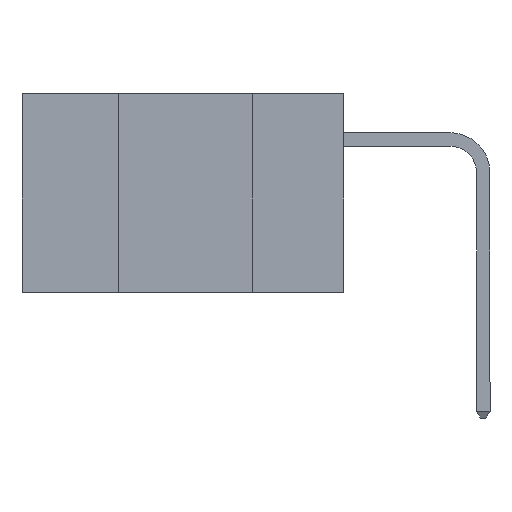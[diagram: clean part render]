
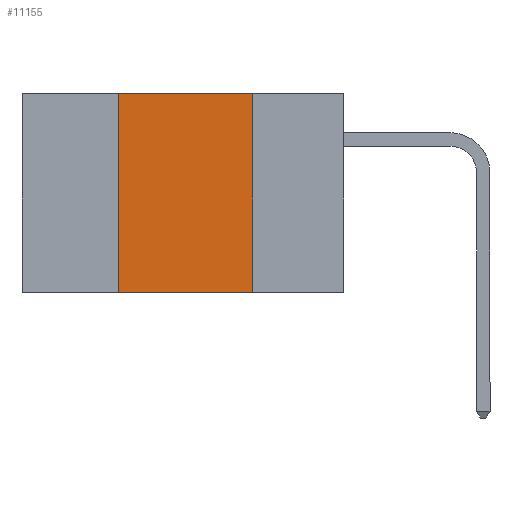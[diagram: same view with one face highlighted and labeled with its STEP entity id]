
A CAD part, left-side view. The second image highlights one B-rep face of the part: STEP entity #11155.
In plain terms, the highlighted planar face has unit normal (-1, 0, 0).
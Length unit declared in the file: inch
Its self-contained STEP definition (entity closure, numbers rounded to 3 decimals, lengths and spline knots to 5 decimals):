
#25 = VECTOR ( 'NONE', #2915, 39.37008 ) ;
#206 = ORIENTED_EDGE ( 'NONE', *, *, #9290, .T. ) ;
#364 = CARTESIAN_POINT ( 'NONE',  ( 0., 0.42, -0.37 ) ) ;
#1461 = DIRECTION ( 'NONE',  ( 0., 0., 1. ) ) ;
#1972 = PLANE ( 'NONE',  #8002 ) ;
#2119 = CARTESIAN_POINT ( 'NONE',  ( 0., 0.42, 0. ) ) ;
#2573 = LINE ( 'NONE', #13075, #5577 ) ;
#2915 = DIRECTION ( 'NONE',  ( 0., 0., -1. ) ) ;
#3255 = DIRECTION ( 'NONE',  ( 1., 0., 0. ) ) ;
#3504 = FACE_OUTER_BOUND ( 'NONE', #11073, .T. ) ;
#3637 = ORIENTED_EDGE ( 'NONE', *, *, #10864, .F. ) ;
#4754 = ORIENTED_EDGE ( 'NONE', *, *, #11659, .F. ) ;
#5577 = VECTOR ( 'NONE', #15518, 39.37008 ) ;
#8002 = AXIS2_PLACEMENT_3D ( 'NONE', #10752, #3255, #11915 ) ;
#8696 = VERTEX_POINT ( 'NONE', #364 ) ;
#9224 = CARTESIAN_POINT ( 'NONE',  ( 0., 0.17, 0. ) ) ;
#9290 = EDGE_CURVE ( 'NONE', #8696, #14213, #11735, .T. ) ;
#9798 = LINE ( 'NONE', #9224, #25 ) ;
#9907 = VERTEX_POINT ( 'NONE', #10927 ) ;
#10333 = ORIENTED_EDGE ( 'NONE', *, *, #14734, .F. ) ;
#10388 = VECTOR ( 'NONE', #1461, 39.37008 ) ;
#10752 = CARTESIAN_POINT ( 'NONE',  ( 0., 0.6, 0. ) ) ;
#10864 = EDGE_CURVE ( 'NONE', #8696, #13258, #13880, .T. ) ;
#10927 = CARTESIAN_POINT ( 'NONE',  ( 0., 0.17, 0. ) ) ;
#11073 = EDGE_LOOP ( 'NONE', ( #4754, #10333, #3637, #206 ) ) ;
#11155 = ADVANCED_FACE ( 'NONE', ( #3504 ), #1972, .F. ) ;
#11659 = EDGE_CURVE ( 'NONE', #9907, #14213, #9798, .T. ) ;
#11735 = LINE ( 'NONE', #12926, #14499 ) ;
#11915 = DIRECTION ( 'NONE',  ( 0., 0., -1. ) ) ;
#12926 = CARTESIAN_POINT ( 'NONE',  ( 0., 0.6, -0.37 ) ) ;
#13075 = CARTESIAN_POINT ( 'NONE',  ( 0., 0.6, 0. ) ) ;
#13258 = VERTEX_POINT ( 'NONE', #2119 ) ;
#13788 = CARTESIAN_POINT ( 'NONE',  ( 0., 0.42, 0. ) ) ;
#13797 = CARTESIAN_POINT ( 'NONE',  ( 0., 0.17, -0.37 ) ) ;
#13880 = LINE ( 'NONE', #13788, #10388 ) ;
#14213 = VERTEX_POINT ( 'NONE', #13797 ) ;
#14499 = VECTOR ( 'NONE', #15355, 39.37008 ) ;
#14734 = EDGE_CURVE ( 'NONE', #13258, #9907, #2573, .T. ) ;
#15355 = DIRECTION ( 'NONE',  ( 0., -1., 0. ) ) ;
#15518 = DIRECTION ( 'NONE',  ( 0., -1., 0. ) ) ;
